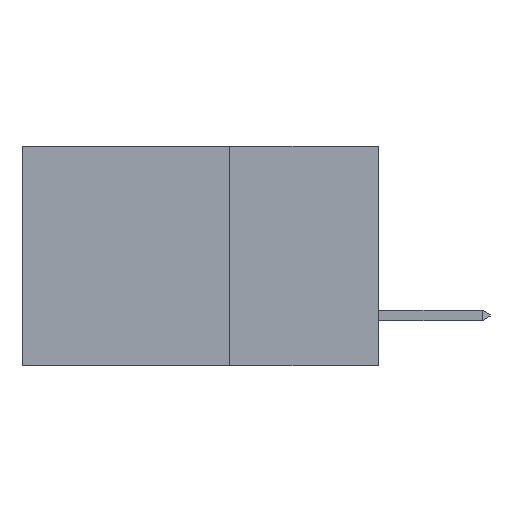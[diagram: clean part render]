
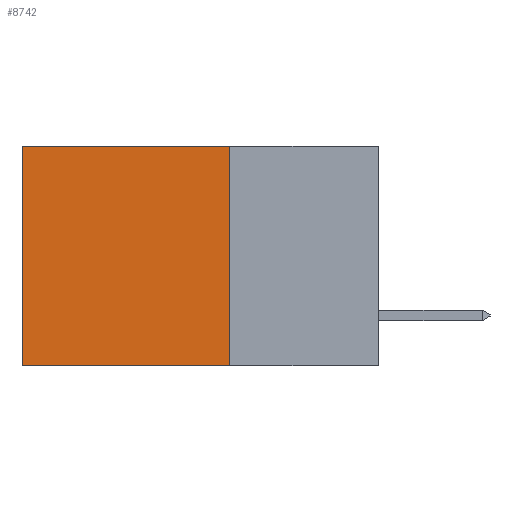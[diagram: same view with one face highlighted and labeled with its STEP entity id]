
A CAD part, left-side view. The second image highlights one B-rep face of the part: STEP entity #8742.
In plain terms, the highlighted planar face has unit normal (-1, 0, 0).
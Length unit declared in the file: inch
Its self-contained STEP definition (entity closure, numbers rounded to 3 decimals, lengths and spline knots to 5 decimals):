
#347 = DIRECTION ( 'NONE',  ( 0., 0., -1. ) ) ;
#393 = EDGE_LOOP ( 'NONE', ( #13590, #6792, #8457, #14314 ) ) ;
#461 = AXIS2_PLACEMENT_3D ( 'NONE', #3046, #8685, #347 ) ;
#586 = VERTEX_POINT ( 'NONE', #13862 ) ;
#1551 = LINE ( 'NONE', #13639, #4372 ) ;
#2375 = VECTOR ( 'NONE', #7659, 39.37008 ) ;
#2568 = EDGE_CURVE ( 'NONE', #7304, #15998, #13515, .T. ) ;
#3046 = CARTESIAN_POINT ( 'NONE',  ( 0.2615, 0.25, -0.37 ) ) ;
#3223 = EDGE_CURVE ( 'NONE', #17938, #586, #9778, .T. ) ;
#3284 = EDGE_CURVE ( 'NONE', #17938, #7304, #9330, .T. ) ;
#4372 = VECTOR ( 'NONE', #6645, 39.37008 ) ;
#6473 = VECTOR ( 'NONE', #16174, 39.37008 ) ;
#6645 = DIRECTION ( 'NONE',  ( 0., 1., 0. ) ) ;
#6792 = ORIENTED_EDGE ( 'NONE', *, *, #9752, .F. ) ;
#6798 = DIRECTION ( 'NONE',  ( 0., 1., 0. ) ) ;
#6860 = CARTESIAN_POINT ( 'NONE',  ( 0.2615, 0.25, 0. ) ) ;
#7304 = VERTEX_POINT ( 'NONE', #15579 ) ;
#7659 = DIRECTION ( 'NONE',  ( 0., 0., -1. ) ) ;
#7968 = CARTESIAN_POINT ( 'NONE',  ( 0.2615, 0.25, -0.37 ) ) ;
#8394 = CARTESIAN_POINT ( 'NONE',  ( 0.2615, 0.25, 0. ) ) ;
#8457 = ORIENTED_EDGE ( 'NONE', *, *, #3223, .F. ) ;
#8685 = DIRECTION ( 'NONE',  ( 1., 0., 0. ) ) ;
#8742 = ADVANCED_FACE ( 'NONE', ( #14488 ), #17107, .F. ) ;
#8897 = VECTOR ( 'NONE', #6798, 39.37008 ) ;
#9330 = LINE ( 'NONE', #6860, #8897 ) ;
#9752 = EDGE_CURVE ( 'NONE', #586, #15998, #1551, .T. ) ;
#9778 = LINE ( 'NONE', #7968, #2375 ) ;
#13515 = LINE ( 'NONE', #16210, #6473 ) ;
#13590 = ORIENTED_EDGE ( 'NONE', *, *, #2568, .T. ) ;
#13639 = CARTESIAN_POINT ( 'NONE',  ( 0.2615, 0.25, -0.37 ) ) ;
#13862 = CARTESIAN_POINT ( 'NONE',  ( 0.2615, 0.25, -0.37 ) ) ;
#14314 = ORIENTED_EDGE ( 'NONE', *, *, #3284, .T. ) ;
#14488 = FACE_OUTER_BOUND ( 'NONE', #393, .T. ) ;
#15579 = CARTESIAN_POINT ( 'NONE',  ( 0.2615, 0.6, 0. ) ) ;
#15998 = VERTEX_POINT ( 'NONE', #17018 ) ;
#16174 = DIRECTION ( 'NONE',  ( 0., 0., -1. ) ) ;
#16210 = CARTESIAN_POINT ( 'NONE',  ( 0.2615, 0.6, -0.37 ) ) ;
#17018 = CARTESIAN_POINT ( 'NONE',  ( 0.2615, 0.6, -0.37 ) ) ;
#17107 = PLANE ( 'NONE',  #461 ) ;
#17938 = VERTEX_POINT ( 'NONE', #8394 ) ;
